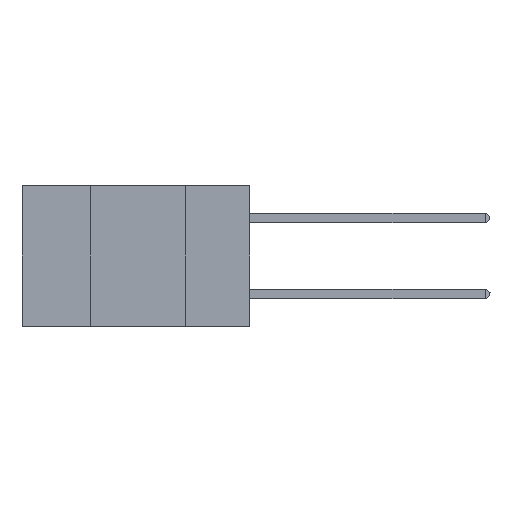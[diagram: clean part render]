
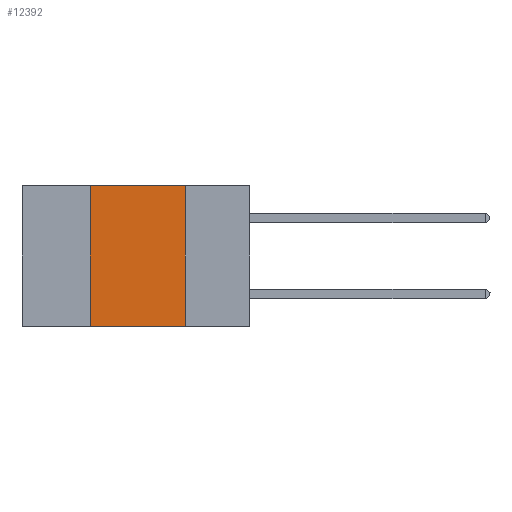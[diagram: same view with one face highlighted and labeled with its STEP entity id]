
A CAD part, left-side view. The second image highlights one B-rep face of the part: STEP entity #12392.
In plain terms, the highlighted planar face has unit normal (-1, 0, 0).
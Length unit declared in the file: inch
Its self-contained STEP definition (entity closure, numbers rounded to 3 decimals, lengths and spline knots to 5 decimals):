
#660 = VECTOR ( 'NONE', #24312, 39.37008 ) ;
#1864 = CARTESIAN_POINT ( 'NONE',  ( 0., 0.6, 0. ) ) ;
#2407 = ORIENTED_EDGE ( 'NONE', *, *, #18234, .F. ) ;
#2790 = CARTESIAN_POINT ( 'NONE',  ( 0., 0.17, -0.37 ) ) ;
#2970 = CARTESIAN_POINT ( 'NONE',  ( 0., 0.6, -0.37 ) ) ;
#3657 = EDGE_CURVE ( 'NONE', #11240, #28009, #14234, .T. ) ;
#4777 = FACE_OUTER_BOUND ( 'NONE', #13492, .T. ) ;
#5374 = VECTOR ( 'NONE', #23134, 39.37008 ) ;
#5698 = CARTESIAN_POINT ( 'NONE',  ( 0., 0.17, 0. ) ) ;
#8949 = VERTEX_POINT ( 'NONE', #2790 ) ;
#8989 = EDGE_CURVE ( 'NONE', #11240, #8949, #16105, .T. ) ;
#10738 = PLANE ( 'NONE',  #23363 ) ;
#11240 = VERTEX_POINT ( 'NONE', #12675 ) ;
#12392 = ADVANCED_FACE ( 'NONE', ( #4777 ), #10738, .F. ) ;
#12675 = CARTESIAN_POINT ( 'NONE',  ( 0., 0.42, -0.37 ) ) ;
#12697 = CARTESIAN_POINT ( 'NONE',  ( 0., 0.42, 0. ) ) ;
#13344 = CARTESIAN_POINT ( 'NONE',  ( 0., 0.17, 0. ) ) ;
#13492 = EDGE_LOOP ( 'NONE', ( #2407, #24699, #13558, #15185 ) ) ;
#13558 = ORIENTED_EDGE ( 'NONE', *, *, #3657, .F. ) ;
#13606 = VERTEX_POINT ( 'NONE', #5698 ) ;
#14234 = LINE ( 'NONE', #20747, #24557 ) ;
#14819 = LINE ( 'NONE', #13344, #660 ) ;
#15185 = ORIENTED_EDGE ( 'NONE', *, *, #8989, .T. ) ;
#16105 = LINE ( 'NONE', #2970, #5374 ) ;
#16950 = CARTESIAN_POINT ( 'NONE',  ( 0., 0.6, 0. ) ) ;
#18234 = EDGE_CURVE ( 'NONE', #13606, #8949, #14819, .T. ) ;
#19980 = EDGE_CURVE ( 'NONE', #28009, #13606, #22607, .T. ) ;
#20747 = CARTESIAN_POINT ( 'NONE',  ( 0., 0.42, 0. ) ) ;
#22607 = LINE ( 'NONE', #16950, #24703 ) ;
#23134 = DIRECTION ( 'NONE',  ( 0., -1., 0. ) ) ;
#23269 = DIRECTION ( 'NONE',  ( 0., -1., 0. ) ) ;
#23363 = AXIS2_PLACEMENT_3D ( 'NONE', #1864, #26385, #26197 ) ;
#24312 = DIRECTION ( 'NONE',  ( 0., 0., -1. ) ) ;
#24557 = VECTOR ( 'NONE', #25021, 39.37008 ) ;
#24699 = ORIENTED_EDGE ( 'NONE', *, *, #19980, .F. ) ;
#24703 = VECTOR ( 'NONE', #23269, 39.37008 ) ;
#25021 = DIRECTION ( 'NONE',  ( 0., 0., 1. ) ) ;
#26197 = DIRECTION ( 'NONE',  ( 0., 0., -1. ) ) ;
#26385 = DIRECTION ( 'NONE',  ( 1., 0., 0. ) ) ;
#28009 = VERTEX_POINT ( 'NONE', #12697 ) ;
